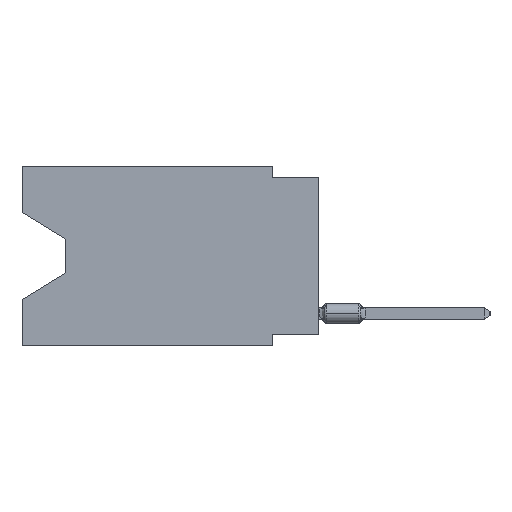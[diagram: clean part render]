
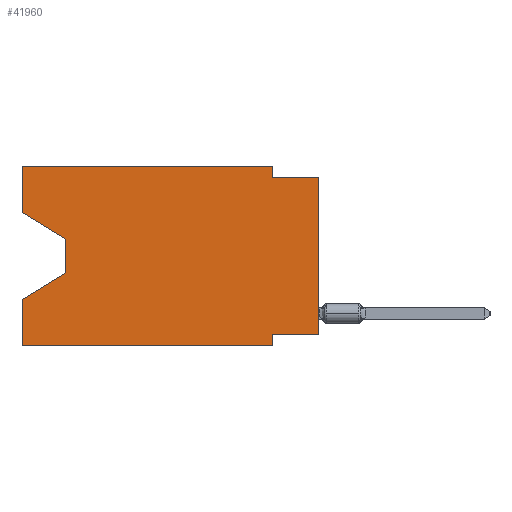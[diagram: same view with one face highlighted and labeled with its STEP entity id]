
A CAD part, left-side view. The second image highlights one B-rep face of the part: STEP entity #41960.
In plain terms, the highlighted planar face has unit normal (-1, 0, 0).
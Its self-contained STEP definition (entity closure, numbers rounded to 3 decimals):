
#213 = VERTEX_POINT ( 'NONE', #20795 ) ;
#697 = EDGE_CURVE ( 'NONE', #34842, #6982, #40242, .T. ) ;
#1095 = CARTESIAN_POINT ( 'NONE',  ( 0., 16.383, 0. ) ) ;
#1463 = CARTESIAN_POINT ( 'NONE',  ( 0., 2.54, -9.906 ) ) ;
#2859 = VERTEX_POINT ( 'NONE', #42288 ) ;
#3332 = CARTESIAN_POINT ( 'NONE',  ( 0., 2.54, -9.271 ) ) ;
#4086 = LINE ( 'NONE', #36678, #28532 ) ;
#4271 = EDGE_CURVE ( 'NONE', #32175, #40711, #19904, .T. ) ;
#4621 = VECTOR ( 'NONE', #30305, 1000. ) ;
#4927 = LINE ( 'NONE', #34692, #27752 ) ;
#5592 = CARTESIAN_POINT ( 'NONE',  ( 0., 0., -0.635 ) ) ;
#5974 = ORIENTED_EDGE ( 'NONE', *, *, #40846, .T. ) ;
#6370 = VECTOR ( 'NONE', #20320, 1000. ) ;
#6982 = VERTEX_POINT ( 'NONE', #3332 ) ;
#7299 = DIRECTION ( 'NONE',  ( 0., 0., 1. ) ) ;
#7636 = VERTEX_POINT ( 'NONE', #1463 ) ;
#7730 = LINE ( 'NONE', #21026, #7801 ) ;
#7801 = VECTOR ( 'NONE', #14267, 1000. ) ;
#8100 = EDGE_CURVE ( 'NONE', #33093, #11391, #41367, .T. ) ;
#8235 = VECTOR ( 'NONE', #12947, 1000. ) ;
#10588 = DIRECTION ( 'NONE',  ( 0., -0.855, -0.519 ) ) ;
#11391 = VERTEX_POINT ( 'NONE', #1095 ) ;
#11631 = CARTESIAN_POINT ( 'NONE',  ( 0., 16.383, 0. ) ) ;
#12191 = VERTEX_POINT ( 'NONE', #41518 ) ;
#12433 = DIRECTION ( 'NONE',  ( 0., 0., -1. ) ) ;
#12947 = DIRECTION ( 'NONE',  ( 0., 0.855, -0.519 ) ) ;
#13150 = ORIENTED_EDGE ( 'NONE', *, *, #8100, .F. ) ;
#13540 = ORIENTED_EDGE ( 'NONE', *, *, #37483, .T. ) ;
#13795 = EDGE_CURVE ( 'NONE', #2859, #22039, #22585, .T. ) ;
#13859 = CARTESIAN_POINT ( 'NONE',  ( 0., 0., -0.635 ) ) ;
#14114 = VECTOR ( 'NONE', #29161, 1000. ) ;
#14267 = DIRECTION ( 'NONE',  ( 0., 0., -1. ) ) ;
#14286 = ORIENTED_EDGE ( 'NONE', *, *, #32399, .T. ) ;
#14533 = EDGE_CURVE ( 'NONE', #213, #2859, #4927, .T. ) ;
#15478 = DIRECTION ( 'NONE',  ( 1., 0., 0. ) ) ;
#15712 = ORIENTED_EDGE ( 'NONE', *, *, #20223, .F. ) ;
#15725 = LINE ( 'NONE', #25533, #16228 ) ;
#16228 = VECTOR ( 'NONE', #29005, 1000. ) ;
#16309 = LINE ( 'NONE', #22652, #22247 ) ;
#17115 = ORIENTED_EDGE ( 'NONE', *, *, #21502, .F. ) ;
#17141 = ORIENTED_EDGE ( 'NONE', *, *, #26503, .T. ) ;
#17390 = CARTESIAN_POINT ( 'NONE',  ( 0., 0., -9.271 ) ) ;
#17569 = DIRECTION ( 'NONE',  ( 0., -1., 0. ) ) ;
#17688 = ORIENTED_EDGE ( 'NONE', *, *, #13795, .F. ) ;
#18287 = VERTEX_POINT ( 'NONE', #35278 ) ;
#18450 = ORIENTED_EDGE ( 'NONE', *, *, #4271, .T. ) ;
#19390 = CARTESIAN_POINT ( 'NONE',  ( 0., 16.383, 0. ) ) ;
#19690 = ORIENTED_EDGE ( 'NONE', *, *, #19819, .F. ) ;
#19819 = EDGE_CURVE ( 'NONE', #11391, #213, #40053, .T. ) ;
#19904 = LINE ( 'NONE', #42665, #8235 ) ;
#19988 = CARTESIAN_POINT ( 'NONE',  ( 0., 16.383, -7.36 ) ) ;
#20223 = EDGE_CURVE ( 'NONE', #6982, #7636, #7730, .T. ) ;
#20320 = DIRECTION ( 'NONE',  ( 0., -1., 0. ) ) ;
#20795 = CARTESIAN_POINT ( 'NONE',  ( 0., 2.54, 0. ) ) ;
#21026 = CARTESIAN_POINT ( 'NONE',  ( 0., 2.54, -9.906 ) ) ;
#21502 = EDGE_CURVE ( 'NONE', #12191, #40711, #29793, .T. ) ;
#21788 = ORIENTED_EDGE ( 'NONE', *, *, #697, .F. ) ;
#22039 = VERTEX_POINT ( 'NONE', #13859 ) ;
#22247 = VECTOR ( 'NONE', #35851, 1000. ) ;
#22465 = FACE_OUTER_BOUND ( 'NONE', #41593, .T. ) ;
#22585 = LINE ( 'NONE', #5592, #24550 ) ;
#22652 = CARTESIAN_POINT ( 'NONE',  ( 0., 0., 0. ) ) ;
#23595 = CARTESIAN_POINT ( 'NONE',  ( 0., 16.383, 0. ) ) ;
#24550 = VECTOR ( 'NONE', #42698, 1000. ) ;
#25533 = CARTESIAN_POINT ( 'NONE',  ( 0., 13.97, -4.013 ) ) ;
#26503 = EDGE_CURVE ( 'NONE', #18287, #32175, #15725, .T. ) ;
#26763 = CARTESIAN_POINT ( 'NONE',  ( 0., 16.383, 0. ) ) ;
#27618 = VECTOR ( 'NONE', #7299, 1000. ) ;
#27752 = VECTOR ( 'NONE', #40991, 1000. ) ;
#28532 = VECTOR ( 'NONE', #17569, 1000. ) ;
#29005 = DIRECTION ( 'NONE',  ( 0., 0., -1. ) ) ;
#29161 = DIRECTION ( 'NONE',  ( 0., 0., 1. ) ) ;
#29793 = LINE ( 'NONE', #26763, #14114 ) ;
#30305 = DIRECTION ( 'NONE',  ( 0., 1., 0. ) ) ;
#30819 = CARTESIAN_POINT ( 'NONE',  ( 0., 16.383, -2.546 ) ) ;
#32175 = VERTEX_POINT ( 'NONE', #33935 ) ;
#32295 = ORIENTED_EDGE ( 'NONE', *, *, #14533, .F. ) ;
#32399 = EDGE_CURVE ( 'NONE', #33093, #18287, #33837, .T. ) ;
#33093 = VERTEX_POINT ( 'NONE', #41542 ) ;
#33837 = LINE ( 'NONE', #30819, #35176 ) ;
#33935 = CARTESIAN_POINT ( 'NONE',  ( 0., 13.97, -5.893 ) ) ;
#34692 = CARTESIAN_POINT ( 'NONE',  ( 0., 2.54, 0. ) ) ;
#34842 = VERTEX_POINT ( 'NONE', #17390 ) ;
#35176 = VECTOR ( 'NONE', #10588, 1000. ) ;
#35278 = CARTESIAN_POINT ( 'NONE',  ( 0., 13.97, -4.013 ) ) ;
#35851 = DIRECTION ( 'NONE',  ( 0., 0., 1. ) ) ;
#36678 = CARTESIAN_POINT ( 'NONE',  ( 0., 16.383, -9.906 ) ) ;
#37483 = EDGE_CURVE ( 'NONE', #34842, #22039, #16309, .T. ) ;
#39348 = PLANE ( 'NONE',  #41714 ) ;
#40053 = LINE ( 'NONE', #23595, #6370 ) ;
#40242 = LINE ( 'NONE', #40454, #4621 ) ;
#40454 = CARTESIAN_POINT ( 'NONE',  ( 0., 0., -9.271 ) ) ;
#40711 = VERTEX_POINT ( 'NONE', #19988 ) ;
#40846 = EDGE_CURVE ( 'NONE', #12191, #7636, #4086, .T. ) ;
#40991 = DIRECTION ( 'NONE',  ( 0., 0., -1. ) ) ;
#41367 = LINE ( 'NONE', #11631, #27618 ) ;
#41518 = CARTESIAN_POINT ( 'NONE',  ( 0., 16.383, -9.906 ) ) ;
#41542 = CARTESIAN_POINT ( 'NONE',  ( 0., 16.383, -2.546 ) ) ;
#41593 = EDGE_LOOP ( 'NONE', ( #14286, #17141, #18450, #17115, #5974, #15712, #21788, #13540, #17688, #32295, #19690, #13150 ) ) ;
#41714 = AXIS2_PLACEMENT_3D ( 'NONE', #19390, #15478, #12433 ) ;
#41960 = ADVANCED_FACE ( 'NONE', ( #22465 ), #39348, .F. ) ;
#42288 = CARTESIAN_POINT ( 'NONE',  ( 0., 2.54, -0.635 ) ) ;
#42665 = CARTESIAN_POINT ( 'NONE',  ( 0., 13.97, -5.893 ) ) ;
#42698 = DIRECTION ( 'NONE',  ( 0., -1., 0. ) ) ;
